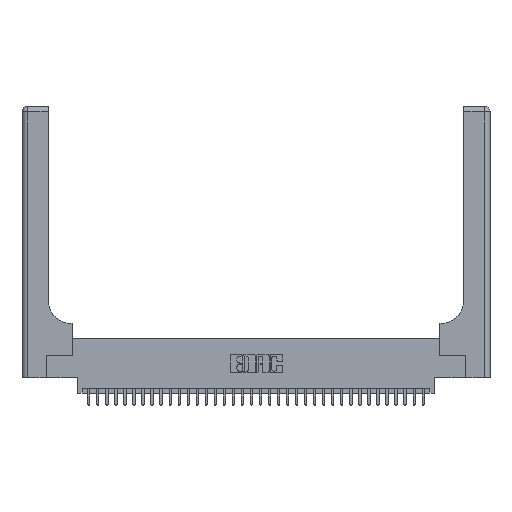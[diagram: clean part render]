
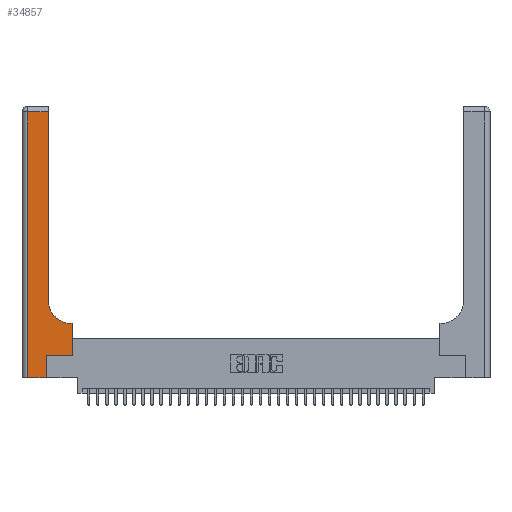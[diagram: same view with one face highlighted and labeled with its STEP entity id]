
A CAD part, top view. The second image highlights one B-rep face of the part: STEP entity #34857.
In plain terms, the highlighted planar face has unit normal (0, 0, 1).
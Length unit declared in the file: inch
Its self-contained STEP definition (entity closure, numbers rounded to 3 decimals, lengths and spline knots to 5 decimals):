
#353 = CARTESIAN_POINT ( 'NONE',  ( 0.5585, 0.25, 0.37 ) ) ;
#642 = CARTESIAN_POINT ( 'NONE',  ( 0., 0., 0.37 ) ) ;
#1525 = CARTESIAN_POINT ( 'NONE',  ( 0.269, 0.25, 0.37 ) ) ;
#1657 = AXIS2_PLACEMENT_3D ( 'NONE', #31179, #14662, #33955 ) ;
#2348 = EDGE_LOOP ( 'NONE', ( #32501, #7879, #15191, #31924, #6821, #33933, #11455, #11057, #20824 ) ) ;
#3194 = CARTESIAN_POINT ( 'NONE',  ( 0.269, 0., 0.37 ) ) ;
#3635 = CARTESIAN_POINT ( 'NONE',  ( 0.5415, 0.6, 0.37 ) ) ;
#3831 = CARTESIAN_POINT ( 'NONE',  ( 0.2915, 0.85, 0.37 ) ) ;
#4235 = CIRCLE ( 'NONE', #1657, 0.25 ) ;
#5393 = CARTESIAN_POINT ( 'NONE',  ( 0.5585, 0.25, 0.37 ) ) ;
#5413 = EDGE_CURVE ( 'NONE', #25953, #7379, #30024, .T. ) ;
#5854 = EDGE_CURVE ( 'NONE', #23747, #7594, #9729, .T. ) ;
#5870 = CARTESIAN_POINT ( 'NONE',  ( 0.06, 2.94, 0.37 ) ) ;
#6139 = VECTOR ( 'NONE', #22497, 39.37008 ) ;
#6451 = VECTOR ( 'NONE', #18492, 39.37008 ) ;
#6624 = LINE ( 'NONE', #18693, #13111 ) ;
#6637 = DIRECTION ( 'NONE',  ( 0., 0., -1. ) ) ;
#6821 = ORIENTED_EDGE ( 'NONE', *, *, #20831, .T. ) ;
#7379 = VERTEX_POINT ( 'NONE', #27146 ) ;
#7594 = VERTEX_POINT ( 'NONE', #31207 ) ;
#7879 = ORIENTED_EDGE ( 'NONE', *, *, #27110, .T. ) ;
#8836 = VERTEX_POINT ( 'NONE', #11595 ) ;
#8919 = VERTEX_POINT ( 'NONE', #3635 ) ;
#9729 = LINE ( 'NONE', #353, #30863 ) ;
#10925 = FACE_OUTER_BOUND ( 'NONE', #2348, .T. ) ;
#11057 = ORIENTED_EDGE ( 'NONE', *, *, #28115, .T. ) ;
#11455 = ORIENTED_EDGE ( 'NONE', *, *, #5854, .T. ) ;
#11595 = CARTESIAN_POINT ( 'NONE',  ( 0.2915, 2.94, 0.37 ) ) ;
#12414 = DIRECTION ( 'NONE',  ( -1., 0., 0. ) ) ;
#13111 = VECTOR ( 'NONE', #21503, 39.37008 ) ;
#13789 = LINE ( 'NONE', #21291, #6451 ) ;
#14082 = CARTESIAN_POINT ( 'NONE',  ( 0.269, 0.25, 0.37 ) ) ;
#14662 = DIRECTION ( 'NONE',  ( 0., 0., -1. ) ) ;
#15191 = ORIENTED_EDGE ( 'NONE', *, *, #34525, .T. ) ;
#15234 = VERTEX_POINT ( 'NONE', #3831 ) ;
#15352 = VECTOR ( 'NONE', #28249, 39.37008 ) ;
#16106 = EDGE_CURVE ( 'NONE', #8919, #15234, #4235, .T. ) ;
#16606 = CARTESIAN_POINT ( 'NONE',  ( 0.2915, 0.6, 0.37 ) ) ;
#16857 = DIRECTION ( 'NONE',  ( 0., 1., 0. ) ) ;
#18492 = DIRECTION ( 'NONE',  ( 0., 1., 0. ) ) ;
#18693 = CARTESIAN_POINT ( 'NONE',  ( 0.06, 3., 0.37 ) ) ;
#19733 = VECTOR ( 'NONE', #12414, 39.37008 ) ;
#20824 = ORIENTED_EDGE ( 'NONE', *, *, #16106, .T. ) ;
#20831 = EDGE_CURVE ( 'NONE', #7379, #26043, #33739, .T. ) ;
#21291 = CARTESIAN_POINT ( 'NONE',  ( 0.2915, 3., 0.37 ) ) ;
#21503 = DIRECTION ( 'NONE',  ( 0., -1., 0. ) ) ;
#22497 = DIRECTION ( 'NONE',  ( 0., 1., 0. ) ) ;
#23173 = CARTESIAN_POINT ( 'NONE',  ( 0., 3., 0.37 ) ) ;
#23177 = VECTOR ( 'NONE', #27708, 39.37008 ) ;
#23406 = CARTESIAN_POINT ( 'NONE',  ( 0., 2.94, 0.37 ) ) ;
#23747 = VERTEX_POINT ( 'NONE', #5393 ) ;
#25953 = VERTEX_POINT ( 'NONE', #28662 ) ;
#25956 = DIRECTION ( 'NONE',  ( -1., 0., 0. ) ) ;
#26043 = VERTEX_POINT ( 'NONE', #1525 ) ;
#27083 = LINE ( 'NONE', #23406, #19733 ) ;
#27110 = EDGE_CURVE ( 'NONE', #8836, #30242, #27083, .T. ) ;
#27146 = CARTESIAN_POINT ( 'NONE',  ( 0.269, 0., 0.37 ) ) ;
#27306 = VECTOR ( 'NONE', #33384, 39.37008 ) ;
#27708 = DIRECTION ( 'NONE',  ( -1., 0., 0. ) ) ;
#28115 = EDGE_CURVE ( 'NONE', #7594, #8919, #30500, .T. ) ;
#28249 = DIRECTION ( 'NONE',  ( 1., 0., 0. ) ) ;
#28662 = CARTESIAN_POINT ( 'NONE',  ( 0.06, 0., 0.37 ) ) ;
#30024 = LINE ( 'NONE', #642, #15352 ) ;
#30086 = AXIS2_PLACEMENT_3D ( 'NONE', #23173, #6637, #25956 ) ;
#30242 = VERTEX_POINT ( 'NONE', #5870 ) ;
#30500 = LINE ( 'NONE', #16606, #23177 ) ;
#30863 = VECTOR ( 'NONE', #16857, 39.37008 ) ;
#31179 = CARTESIAN_POINT ( 'NONE',  ( 0.5415, 0.85, 0.37 ) ) ;
#31207 = CARTESIAN_POINT ( 'NONE',  ( 0.5585, 0.6, 0.37 ) ) ;
#31924 = ORIENTED_EDGE ( 'NONE', *, *, #5413, .T. ) ;
#32236 = EDGE_CURVE ( 'NONE', #15234, #8836, #13789, .T. ) ;
#32501 = ORIENTED_EDGE ( 'NONE', *, *, #32236, .T. ) ;
#33384 = DIRECTION ( 'NONE',  ( 1., 0., 0. ) ) ;
#33739 = LINE ( 'NONE', #3194, #6139 ) ;
#33755 = LINE ( 'NONE', #14082, #27306 ) ;
#33933 = ORIENTED_EDGE ( 'NONE', *, *, #35277, .T. ) ;
#33955 = DIRECTION ( 'NONE',  ( 1., 0., 0. ) ) ;
#34141 = PLANE ( 'NONE',  #30086 ) ;
#34525 = EDGE_CURVE ( 'NONE', #30242, #25953, #6624, .T. ) ;
#34857 = ADVANCED_FACE ( 'NONE', ( #10925 ), #34141, .F. ) ;
#35277 = EDGE_CURVE ( 'NONE', #26043, #23747, #33755, .T. ) ;
